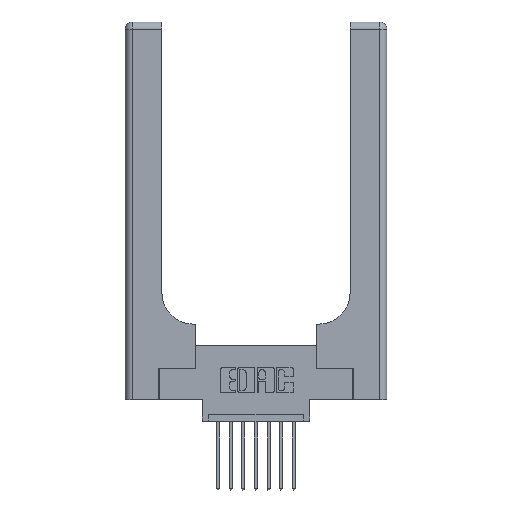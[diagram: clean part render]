
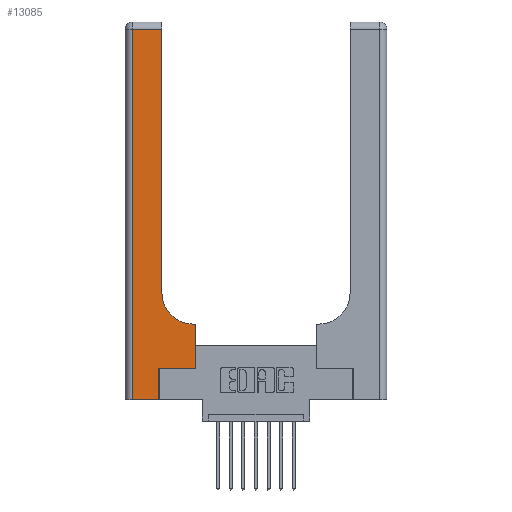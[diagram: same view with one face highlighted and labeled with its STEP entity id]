
A CAD part, top view. The second image highlights one B-rep face of the part: STEP entity #13085.
In plain terms, the highlighted planar face has unit normal (0, 0, 1).
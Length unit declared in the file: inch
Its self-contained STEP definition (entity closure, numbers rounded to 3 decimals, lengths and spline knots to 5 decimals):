
#98 = CARTESIAN_POINT ( 'NONE',  ( 0.269, 0.25, 0.37 ) ) ;
#248 = EDGE_CURVE ( 'NONE', #15234, #12921, #14374, .T. ) ;
#369 = DIRECTION ( 'NONE',  ( 0., 0., -1. ) ) ;
#414 = VECTOR ( 'NONE', #14891, 39.37008 ) ;
#430 = DIRECTION ( 'NONE',  ( 0., 1., 0. ) ) ;
#475 = CARTESIAN_POINT ( 'NONE',  ( 0.2915, 0.85, 0.37 ) ) ;
#573 = DIRECTION ( 'NONE',  ( -1., 0., 0. ) ) ;
#723 = ORIENTED_EDGE ( 'NONE', *, *, #2041, .T. ) ;
#897 = ORIENTED_EDGE ( 'NONE', *, *, #10831, .T. ) ;
#909 = VERTEX_POINT ( 'NONE', #14717 ) ;
#1543 = VECTOR ( 'NONE', #430, 39.37008 ) ;
#1627 = DIRECTION ( 'NONE',  ( -1., 0., 0. ) ) ;
#2041 = EDGE_CURVE ( 'NONE', #13486, #15234, #13218, .T. ) ;
#2114 = LINE ( 'NONE', #14529, #2312 ) ;
#2179 = VERTEX_POINT ( 'NONE', #8609 ) ;
#2183 = EDGE_LOOP ( 'NONE', ( #3136, #3067, #4266, #9242, #2376, #723, #8374, #8967, #897 ) ) ;
#2273 = LINE ( 'NONE', #13546, #1543 ) ;
#2312 = VECTOR ( 'NONE', #7442, 39.37008 ) ;
#2376 = ORIENTED_EDGE ( 'NONE', *, *, #11539, .T. ) ;
#3067 = ORIENTED_EDGE ( 'NONE', *, *, #10017, .T. ) ;
#3136 = ORIENTED_EDGE ( 'NONE', *, *, #10921, .T. ) ;
#3647 = LINE ( 'NONE', #10657, #5295 ) ;
#3886 = CARTESIAN_POINT ( 'NONE',  ( 0.06, 2.94, 0.37 ) ) ;
#3991 = AXIS2_PLACEMENT_3D ( 'NONE', #10988, #369, #1627 ) ;
#4090 = EDGE_CURVE ( 'NONE', #909, #2179, #10602, .T. ) ;
#4266 = ORIENTED_EDGE ( 'NONE', *, *, #13060, .T. ) ;
#4523 = VECTOR ( 'NONE', #4923, 39.37008 ) ;
#4742 = DIRECTION ( 'NONE',  ( 0., 1., 0. ) ) ;
#4923 = DIRECTION ( 'NONE',  ( 1., 0., 0. ) ) ;
#5082 = VECTOR ( 'NONE', #9276, 39.37008 ) ;
#5295 = VECTOR ( 'NONE', #4742, 39.37008 ) ;
#5497 = CARTESIAN_POINT ( 'NONE',  ( 0.2915, 2.94, 0.37 ) ) ;
#5868 = CARTESIAN_POINT ( 'NONE',  ( 0.2915, 0.6, 0.37 ) ) ;
#7442 = DIRECTION ( 'NONE',  ( 0., -1., 0. ) ) ;
#7637 = CARTESIAN_POINT ( 'NONE',  ( 0., 2.94, 0.37 ) ) ;
#7676 = LINE ( 'NONE', #5868, #5082 ) ;
#8066 = VERTEX_POINT ( 'NONE', #12797 ) ;
#8374 = ORIENTED_EDGE ( 'NONE', *, *, #248, .T. ) ;
#8609 = CARTESIAN_POINT ( 'NONE',  ( 0.269, 0., 0.37 ) ) ;
#8919 = CARTESIAN_POINT ( 'NONE',  ( 0., 0., 0.37 ) ) ;
#8967 = ORIENTED_EDGE ( 'NONE', *, *, #9124, .T. ) ;
#9124 = EDGE_CURVE ( 'NONE', #12921, #8066, #7676, .T. ) ;
#9242 = ORIENTED_EDGE ( 'NONE', *, *, #4090, .T. ) ;
#9276 = DIRECTION ( 'NONE',  ( -1., 0., 0. ) ) ;
#9419 = DIRECTION ( 'NONE',  ( 1., 0., 0. ) ) ;
#9489 = AXIS2_PLACEMENT_3D ( 'NONE', #10438, #11729, #9419 ) ;
#9889 = VECTOR ( 'NONE', #573, 39.37008 ) ;
#9945 = VERTEX_POINT ( 'NONE', #475 ) ;
#10017 = EDGE_CURVE ( 'NONE', #12017, #13031, #14320, .T. ) ;
#10438 = CARTESIAN_POINT ( 'NONE',  ( 0.5415, 0.85, 0.37 ) ) ;
#10516 = CARTESIAN_POINT ( 'NONE',  ( 0.5585, 0.6, 0.37 ) ) ;
#10602 = LINE ( 'NONE', #8919, #414 ) ;
#10657 = CARTESIAN_POINT ( 'NONE',  ( 0.269, 0., 0.37 ) ) ;
#10831 = EDGE_CURVE ( 'NONE', #8066, #9945, #13359, .T. ) ;
#10896 = DIRECTION ( 'NONE',  ( 0., 1., 0. ) ) ;
#10921 = EDGE_CURVE ( 'NONE', #9945, #12017, #2273, .T. ) ;
#10988 = CARTESIAN_POINT ( 'NONE',  ( 0., 3., 0.37 ) ) ;
#11539 = EDGE_CURVE ( 'NONE', #2179, #13486, #3647, .T. ) ;
#11729 = DIRECTION ( 'NONE',  ( 0., 0., -1. ) ) ;
#11957 = CARTESIAN_POINT ( 'NONE',  ( 0.269, 0.25, 0.37 ) ) ;
#12017 = VERTEX_POINT ( 'NONE', #5497 ) ;
#12111 = CARTESIAN_POINT ( 'NONE',  ( 0.5585, 0.25, 0.37 ) ) ;
#12458 = FACE_OUTER_BOUND ( 'NONE', #2183, .T. ) ;
#12797 = CARTESIAN_POINT ( 'NONE',  ( 0.5415, 0.6, 0.37 ) ) ;
#12921 = VERTEX_POINT ( 'NONE', #10516 ) ;
#13031 = VERTEX_POINT ( 'NONE', #3886 ) ;
#13060 = EDGE_CURVE ( 'NONE', #13031, #909, #2114, .T. ) ;
#13085 = ADVANCED_FACE ( 'NONE', ( #12458 ), #13247, .F. ) ;
#13218 = LINE ( 'NONE', #11957, #4523 ) ;
#13247 = PLANE ( 'NONE',  #3991 ) ;
#13359 = CIRCLE ( 'NONE', #9489, 0.25 ) ;
#13486 = VERTEX_POINT ( 'NONE', #98 ) ;
#13546 = CARTESIAN_POINT ( 'NONE',  ( 0.2915, 3., 0.37 ) ) ;
#14167 = CARTESIAN_POINT ( 'NONE',  ( 0.5585, 0.25, 0.37 ) ) ;
#14320 = LINE ( 'NONE', #7637, #9889 ) ;
#14374 = LINE ( 'NONE', #14167, #15291 ) ;
#14529 = CARTESIAN_POINT ( 'NONE',  ( 0.06, 3., 0.37 ) ) ;
#14717 = CARTESIAN_POINT ( 'NONE',  ( 0.06, 0., 0.37 ) ) ;
#14891 = DIRECTION ( 'NONE',  ( 1., 0., 0. ) ) ;
#15234 = VERTEX_POINT ( 'NONE', #12111 ) ;
#15291 = VECTOR ( 'NONE', #10896, 39.37008 ) ;
